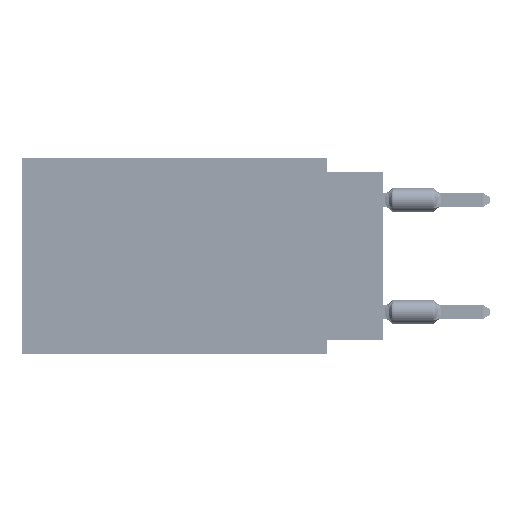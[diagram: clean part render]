
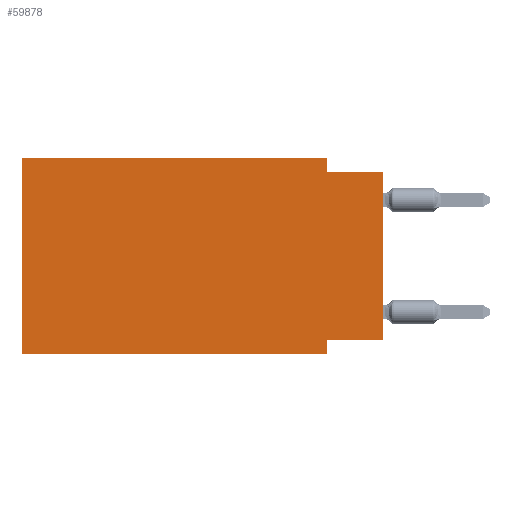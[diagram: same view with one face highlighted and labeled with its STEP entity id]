
A CAD part, left-side view. The second image highlights one B-rep face of the part: STEP entity #59878.
In plain terms, the highlighted planar face has unit normal (-1, 0, 0).
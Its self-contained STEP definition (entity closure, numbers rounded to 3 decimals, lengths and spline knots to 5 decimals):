
#816 = CARTESIAN_POINT ( 'NONE',  ( 0., 0.645, -0.35 ) ) ;
#1426 = VERTEX_POINT ( 'NONE', #89431 ) ;
#1837 = LINE ( 'NONE', #47927, #43473 ) ;
#4590 = ORIENTED_EDGE ( 'NONE', *, *, #13788, .F. ) ;
#5848 = ORIENTED_EDGE ( 'NONE', *, *, #44734, .T. ) ;
#5961 = CARTESIAN_POINT ( 'NONE',  ( 0., 0.645, -0.35 ) ) ;
#7853 = LINE ( 'NONE', #38742, #76023 ) ;
#7990 = DIRECTION ( 'NONE',  ( 0., 0., -1. ) ) ;
#9439 = DIRECTION ( 'NONE',  ( 0., 0., 1. ) ) ;
#10300 = ORIENTED_EDGE ( 'NONE', *, *, #35179, .T. ) ;
#13788 = EDGE_CURVE ( 'NONE', #94332, #33035, #89335, .T. ) ;
#16441 = CARTESIAN_POINT ( 'NONE',  ( 0., 0.645, 0. ) ) ;
#16636 = FACE_OUTER_BOUND ( 'NONE', #18354, .T. ) ;
#16832 = CARTESIAN_POINT ( 'NONE',  ( 0., 0.1, -0.325 ) ) ;
#16863 = ORIENTED_EDGE ( 'NONE', *, *, #19820, .F. ) ;
#18354 = EDGE_LOOP ( 'NONE', ( #5848, #23359, #53023, #75239, #71938, #10300, #16863, #4590 ) ) ;
#19820 = EDGE_CURVE ( 'NONE', #33035, #95992, #30775, .T. ) ;
#21637 = DIRECTION ( 'NONE',  ( 0., -1., 0. ) ) ;
#23282 = EDGE_CURVE ( 'NONE', #1426, #83216, #52449, .T. ) ;
#23359 = ORIENTED_EDGE ( 'NONE', *, *, #89496, .F. ) ;
#24509 = DIRECTION ( 'NONE',  ( 0., 0., 1. ) ) ;
#25037 = DIRECTION ( 'NONE',  ( 0., 0., -1. ) ) ;
#27378 = VECTOR ( 'NONE', #91440, 39.37008 ) ;
#29226 = LINE ( 'NONE', #5961, #86984 ) ;
#29510 = AXIS2_PLACEMENT_3D ( 'NONE', #61216, #93121, #62713 ) ;
#30775 = LINE ( 'NONE', #37893, #53107 ) ;
#33035 = VERTEX_POINT ( 'NONE', #16832 ) ;
#34222 = DIRECTION ( 'NONE',  ( 0., -1., 0. ) ) ;
#35179 = EDGE_CURVE ( 'NONE', #54344, #95992, #29226, .T. ) ;
#37893 = CARTESIAN_POINT ( 'NONE',  ( 0., 0.1, -0.35 ) ) ;
#38742 = CARTESIAN_POINT ( 'NONE',  ( 0., 0.1, 0. ) ) ;
#39761 = EDGE_CURVE ( 'NONE', #54344, #1426, #48320, .T. ) ;
#40191 = VERTEX_POINT ( 'NONE', #54683 ) ;
#43473 = VECTOR ( 'NONE', #9439, 39.37008 ) ;
#43517 = CARTESIAN_POINT ( 'NONE',  ( 0., 0., -0.025 ) ) ;
#44734 = EDGE_CURVE ( 'NONE', #94332, #84266, #1837, .T. ) ;
#47927 = CARTESIAN_POINT ( 'NONE',  ( 0., 0., 0. ) ) ;
#48320 = LINE ( 'NONE', #16441, #73557 ) ;
#49169 = CARTESIAN_POINT ( 'NONE',  ( 0., 0.1, -0.35 ) ) ;
#49707 = CARTESIAN_POINT ( 'NONE',  ( 0., 0., -0.325 ) ) ;
#52449 = LINE ( 'NONE', #84809, #27378 ) ;
#53023 = ORIENTED_EDGE ( 'NONE', *, *, #97637, .F. ) ;
#53107 = VECTOR ( 'NONE', #7990, 39.37008 ) ;
#53665 = VECTOR ( 'NONE', #90347, 39.37008 ) ;
#54137 = PLANE ( 'NONE',  #29510 ) ;
#54344 = VERTEX_POINT ( 'NONE', #816 ) ;
#54683 = CARTESIAN_POINT ( 'NONE',  ( 0., 0.1, -0.025 ) ) ;
#57015 = CARTESIAN_POINT ( 'NONE',  ( 0., 0., -0.025 ) ) ;
#59878 = ADVANCED_FACE ( 'NONE', ( #16636 ), #54137, .F. ) ;
#61216 = CARTESIAN_POINT ( 'NONE',  ( 0., 0.645, 0. ) ) ;
#62364 = VECTOR ( 'NONE', #34222, 39.37008 ) ;
#62713 = DIRECTION ( 'NONE',  ( 0., 0., -1. ) ) ;
#71938 = ORIENTED_EDGE ( 'NONE', *, *, #39761, .F. ) ;
#73206 = LINE ( 'NONE', #57015, #62364 ) ;
#73557 = VECTOR ( 'NONE', #24509, 39.37008 ) ;
#75239 = ORIENTED_EDGE ( 'NONE', *, *, #23282, .F. ) ;
#76023 = VECTOR ( 'NONE', #25037, 39.37008 ) ;
#80732 = CARTESIAN_POINT ( 'NONE',  ( 0., 0., -0.325 ) ) ;
#83216 = VERTEX_POINT ( 'NONE', #99187 ) ;
#84266 = VERTEX_POINT ( 'NONE', #43517 ) ;
#84809 = CARTESIAN_POINT ( 'NONE',  ( 0., 0.645, 0. ) ) ;
#86984 = VECTOR ( 'NONE', #21637, 39.37008 ) ;
#89335 = LINE ( 'NONE', #80732, #53665 ) ;
#89431 = CARTESIAN_POINT ( 'NONE',  ( 0., 0.645, 0. ) ) ;
#89496 = EDGE_CURVE ( 'NONE', #40191, #84266, #73206, .T. ) ;
#90347 = DIRECTION ( 'NONE',  ( 0., 1., 0. ) ) ;
#91440 = DIRECTION ( 'NONE',  ( 0., -1., 0. ) ) ;
#93121 = DIRECTION ( 'NONE',  ( 1., 0., 0. ) ) ;
#94332 = VERTEX_POINT ( 'NONE', #49707 ) ;
#95992 = VERTEX_POINT ( 'NONE', #49169 ) ;
#97637 = EDGE_CURVE ( 'NONE', #83216, #40191, #7853, .T. ) ;
#99187 = CARTESIAN_POINT ( 'NONE',  ( 0., 0.1, 0. ) ) ;
